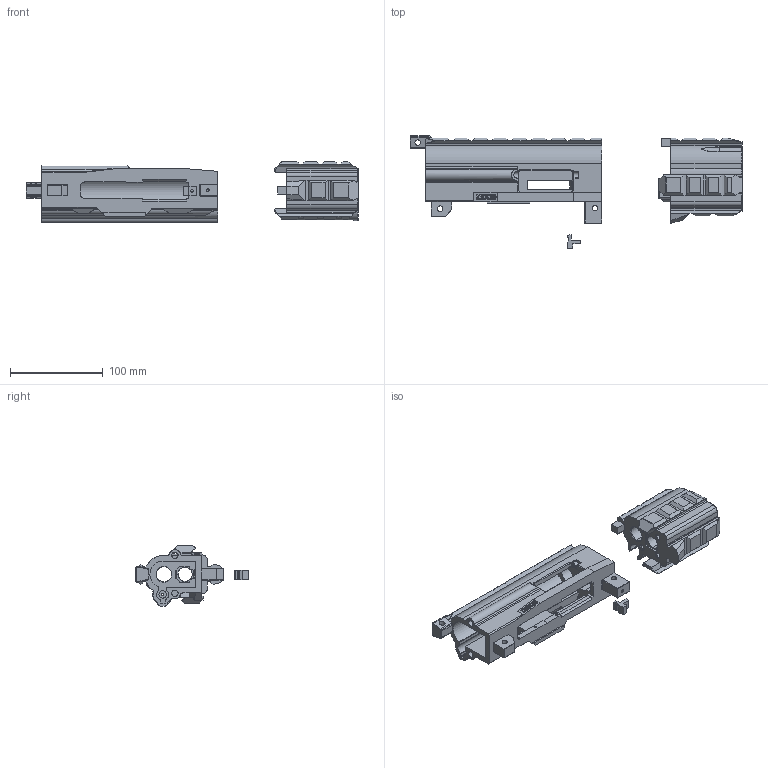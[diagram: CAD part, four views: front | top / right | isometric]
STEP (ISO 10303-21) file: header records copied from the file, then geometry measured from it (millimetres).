
FILE_DESCRIPTION(('STEP AP214'),'1');
FILE_NAME('MOD9 RP9 Set v2.0.stp','2020-10-10T22:22:47',(' '),(' '),'Spatial InterOp 3D',' ',' ');
FILE_SCHEMA(('AUTOMOTIVE_DESIGN { 1 0 10303 214 1 1 1 1 }'));
Length unit declared in the file: metre
Products named in the file (4): MOD9 RP9 Set v2.0; Mod9 RP9 Barrel Retainer Final; Mod9 RP9 Upper Receiver Final; MOD9_RP9_feed_ramp
Assembly tree (3 placements, depth 2):
  MOD9 RP9 Set v2.0
    Mod9 RP9 Barrel Retainer Final
    Mod9 RP9 Upper Receiver Final
    MOD9_RP9_feed_ramp
Bounding box: 358.57 x 121.84 x 65.85 mm (x, y, z)
Volume: 410921.2 mm3; surface area: 137472.4 mm2
Topology: 3 solids, 3 shells, 1233 faces, 3389 edges, 2175 vertices
Faces by surface type: plane 474, cylinder 388, bspline 220, cone 93, torus 36, extrusion 14, sphere 8
Entity records: 43782 total; most frequent: CARTESIAN_POINT 13537, ORIENTED_EDGE 6770, DIRECTION 5614, EDGE_CURVE 3385, VERTEX_POINT 2175, VECTOR 1874, AXIS2_PLACEMENT_3D 1870, LINE 1860
